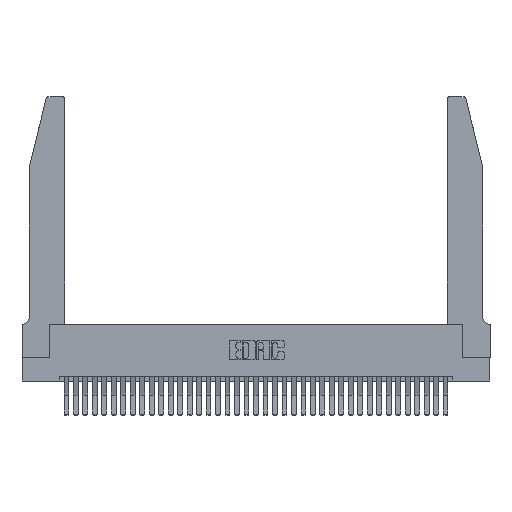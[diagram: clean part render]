
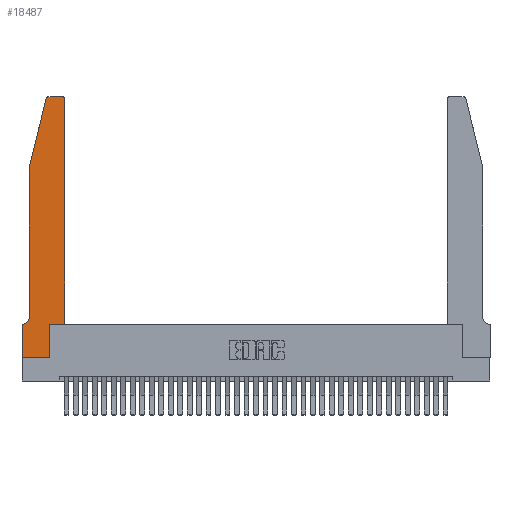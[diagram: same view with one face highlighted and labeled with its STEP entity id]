
A CAD part, top view. The second image highlights one B-rep face of the part: STEP entity #18487.
In plain terms, the highlighted planar face has unit normal (0, 0, 1).
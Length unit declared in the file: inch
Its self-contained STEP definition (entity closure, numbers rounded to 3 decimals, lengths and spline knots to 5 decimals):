
#69 = EDGE_CURVE ( 'NONE', #36676, #17136, #34348, .T. ) ;
#224 = VERTEX_POINT ( 'NONE', #26679 ) ;
#287 = DIRECTION ( 'NONE',  ( 0., 0., -1. ) ) ;
#340 = ORIENTED_EDGE ( 'NONE', *, *, #19087, .T. ) ;
#527 = EDGE_CURVE ( 'NONE', #18967, #36676, #6578, .T. ) ;
#1837 = ORIENTED_EDGE ( 'NONE', *, *, #527, .T. ) ;
#1856 = ORIENTED_EDGE ( 'NONE', *, *, #1985, .T. ) ;
#1975 = CARTESIAN_POINT ( 'NONE',  ( 0.4505, 0.35, 0.37 ) ) ;
#1985 = EDGE_CURVE ( 'NONE', #25116, #20775, #33339, .T. ) ;
#2225 = DIRECTION ( 'NONE',  ( 1., 0., 0. ) ) ;
#3410 = DIRECTION ( 'NONE',  ( 0., 1., 0. ) ) ;
#3851 = ORIENTED_EDGE ( 'NONE', *, *, #35568, .T. ) ;
#5083 = DIRECTION ( 'NONE',  ( -0.239, -0.971, 0. ) ) ;
#5497 = CARTESIAN_POINT ( 'NONE',  ( 0.0755, 2., 0.37 ) ) ;
#5727 = CARTESIAN_POINT ( 'NONE',  ( 0., 0.35, 0.37 ) ) ;
#6361 = LINE ( 'NONE', #14282, #20876 ) ;
#6578 = LINE ( 'NONE', #1975, #27714 ) ;
#6996 = ORIENTED_EDGE ( 'NONE', *, *, #20637, .T. ) ;
#7161 = CARTESIAN_POINT ( 'NONE',  ( 0.0755, 0.42, 0.37 ) ) ;
#7198 = ORIENTED_EDGE ( 'NONE', *, *, #10284, .T. ) ;
#8018 = PLANE ( 'NONE',  #21511 ) ;
#8537 = DIRECTION ( 'NONE',  ( 1., 0., 0. ) ) ;
#8553 = LINE ( 'NONE', #15827, #23876 ) ;
#8865 = CIRCLE ( 'NONE', #21458, 0.07 ) ;
#9119 = EDGE_CURVE ( 'NONE', #35174, #224, #8553, .T. ) ;
#9433 = VERTEX_POINT ( 'NONE', #5727 ) ;
#9565 = EDGE_CURVE ( 'NONE', #224, #22683, #24146, .T. ) ;
#10084 = DIRECTION ( 'NONE',  ( -1., 0., 0. ) ) ;
#10284 = EDGE_CURVE ( 'NONE', #9433, #35174, #16064, .T. ) ;
#10386 = DIRECTION ( 'NONE',  ( 1., 0., 0. ) ) ;
#10434 = DIRECTION ( 'NONE',  ( 0., 0., 1. ) ) ;
#10913 = CARTESIAN_POINT ( 'NONE',  ( 0.284, 2.72, 0.37 ) ) ;
#11249 = CARTESIAN_POINT ( 'NONE',  ( 0., 0., 0.37 ) ) ;
#11261 = DIRECTION ( 'NONE',  ( 0., -1., 0. ) ) ;
#11575 = ORIENTED_EDGE ( 'NONE', *, *, #9565, .T. ) ;
#11736 = EDGE_CURVE ( 'NONE', #32415, #15411, #36758, .T. ) ;
#12309 = EDGE_LOOP ( 'NONE', ( #3851, #32197, #340, #1856, #16196, #6996, #7198, #33823, #11575, #34336, #1837, #19066 ) ) ;
#13189 = AXIS2_PLACEMENT_3D ( 'NONE', #24341, #10434, #10386 ) ;
#13868 = DIRECTION ( 'NONE',  ( 1., 0., 0. ) ) ;
#13955 = LINE ( 'NONE', #19560, #28233 ) ;
#14282 = CARTESIAN_POINT ( 'NONE',  ( 0.4505, 0.35, 0.37 ) ) ;
#15147 = VECTOR ( 'NONE', #21386, 39.37008 ) ;
#15183 = CARTESIAN_POINT ( 'NONE',  ( 0.0755, 0.35, 0.37 ) ) ;
#15411 = VERTEX_POINT ( 'NONE', #33416 ) ;
#15726 = EDGE_CURVE ( 'NONE', #20775, #25629, #8865, .T. ) ;
#15827 = CARTESIAN_POINT ( 'NONE',  ( 0., 0., 0.37 ) ) ;
#16064 = LINE ( 'NONE', #18499, #15147 ) ;
#16196 = ORIENTED_EDGE ( 'NONE', *, *, #15726, .T. ) ;
#16712 = FACE_OUTER_BOUND ( 'NONE', #12309, .T. ) ;
#16783 = CARTESIAN_POINT ( 'NONE',  ( 0., 0.35, 0.37 ) ) ;
#17136 = VERTEX_POINT ( 'NONE', #29913 ) ;
#17768 = CARTESIAN_POINT ( 'NONE',  ( 0.0055, 0.42, 0.37 ) ) ;
#18487 = ADVANCED_FACE ( 'NONE', ( #16712 ), #8018, .T. ) ;
#18499 = CARTESIAN_POINT ( 'NONE',  ( 0., 0., 0.37 ) ) ;
#18967 = VERTEX_POINT ( 'NONE', #24536 ) ;
#19066 = ORIENTED_EDGE ( 'NONE', *, *, #69, .T. ) ;
#19087 = EDGE_CURVE ( 'NONE', #15411, #25116, #13955, .T. ) ;
#19176 = VECTOR ( 'NONE', #11261, 39.37008 ) ;
#19560 = CARTESIAN_POINT ( 'NONE',  ( 0.0755, 2., 0.37 ) ) ;
#19681 = DIRECTION ( 'NONE',  ( 0., 0., 1. ) ) ;
#20637 = EDGE_CURVE ( 'NONE', #25629, #9433, #29422, .T. ) ;
#20666 = DIRECTION ( 'NONE',  ( -1., 0., 0. ) ) ;
#20775 = VERTEX_POINT ( 'NONE', #7161 ) ;
#20876 = VECTOR ( 'NONE', #8537, 39.37008 ) ;
#21386 = DIRECTION ( 'NONE',  ( 0., -1., 0. ) ) ;
#21458 = AXIS2_PLACEMENT_3D ( 'NONE', #17768, #287, #20666 ) ;
#21511 = AXIS2_PLACEMENT_3D ( 'NONE', #16783, #19681, #2225 ) ;
#22378 = CARTESIAN_POINT ( 'NONE',  ( 0.2865, 0.35, 0.37 ) ) ;
#22683 = VERTEX_POINT ( 'NONE', #22378 ) ;
#23876 = VECTOR ( 'NONE', #32818, 39.37008 ) ;
#24146 = LINE ( 'NONE', #32039, #32533 ) ;
#24341 = CARTESIAN_POINT ( 'NONE',  ( 0.4205, 2.72, 0.37 ) ) ;
#24487 = CARTESIAN_POINT ( 'NONE',  ( 0.284, 2.75, 0.37 ) ) ;
#24536 = CARTESIAN_POINT ( 'NONE',  ( 0.4505, 0.35, 0.37 ) ) ;
#25116 = VERTEX_POINT ( 'NONE', #5497 ) ;
#25629 = VERTEX_POINT ( 'NONE', #33415 ) ;
#26679 = CARTESIAN_POINT ( 'NONE',  ( 0.2865, 0., 0.37 ) ) ;
#27303 = VECTOR ( 'NONE', #10084, 39.37008 ) ;
#27714 = VECTOR ( 'NONE', #3410, 39.37008 ) ;
#28233 = VECTOR ( 'NONE', #5083, 39.37008 ) ;
#28432 = CARTESIAN_POINT ( 'NONE',  ( 0.0755, 2., 0.37 ) ) ;
#28697 = AXIS2_PLACEMENT_3D ( 'NONE', #10913, #30922, #13868 ) ;
#29315 = EDGE_CURVE ( 'NONE', #22683, #18967, #6361, .T. ) ;
#29422 = LINE ( 'NONE', #15183, #36031 ) ;
#29478 = DIRECTION ( 'NONE',  ( -1., 0., 0. ) ) ;
#29913 = CARTESIAN_POINT ( 'NONE',  ( 0.4205, 2.75, 0.37 ) ) ;
#30112 = CARTESIAN_POINT ( 'NONE',  ( 0.2605, 2.75, 0.37 ) ) ;
#30922 = DIRECTION ( 'NONE',  ( 0., 0., 1. ) ) ;
#30971 = CARTESIAN_POINT ( 'NONE',  ( 0.4505, 2.72, 0.37 ) ) ;
#32039 = CARTESIAN_POINT ( 'NONE',  ( 0.2865, 0.35, 0.37 ) ) ;
#32197 = ORIENTED_EDGE ( 'NONE', *, *, #11736, .T. ) ;
#32415 = VERTEX_POINT ( 'NONE', #24487 ) ;
#32533 = VECTOR ( 'NONE', #34855, 39.37008 ) ;
#32818 = DIRECTION ( 'NONE',  ( 1., 0., 0. ) ) ;
#33339 = LINE ( 'NONE', #28432, #19176 ) ;
#33415 = CARTESIAN_POINT ( 'NONE',  ( 0.0055, 0.35, 0.37 ) ) ;
#33416 = CARTESIAN_POINT ( 'NONE',  ( 0.25487, 2.72718, 0.37 ) ) ;
#33823 = ORIENTED_EDGE ( 'NONE', *, *, #9119, .T. ) ;
#34336 = ORIENTED_EDGE ( 'NONE', *, *, #29315, .T. ) ;
#34348 = CIRCLE ( 'NONE', #13189, 0.03 ) ;
#34783 = LINE ( 'NONE', #30112, #27303 ) ;
#34855 = DIRECTION ( 'NONE',  ( 0., 1., 0. ) ) ;
#35174 = VERTEX_POINT ( 'NONE', #11249 ) ;
#35568 = EDGE_CURVE ( 'NONE', #17136, #32415, #34783, .T. ) ;
#36031 = VECTOR ( 'NONE', #29478, 39.37008 ) ;
#36676 = VERTEX_POINT ( 'NONE', #30971 ) ;
#36758 = CIRCLE ( 'NONE', #28697, 0.03 ) ;
